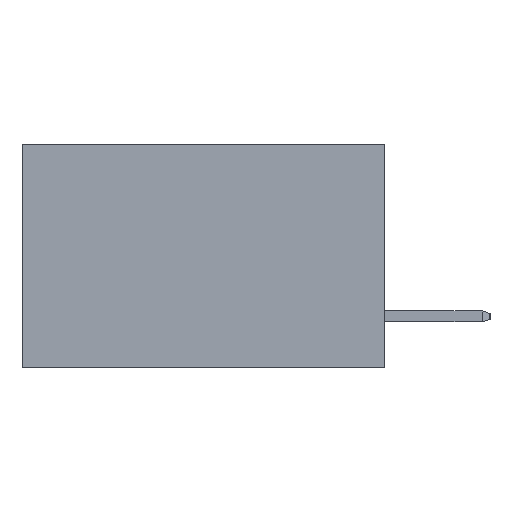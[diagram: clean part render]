
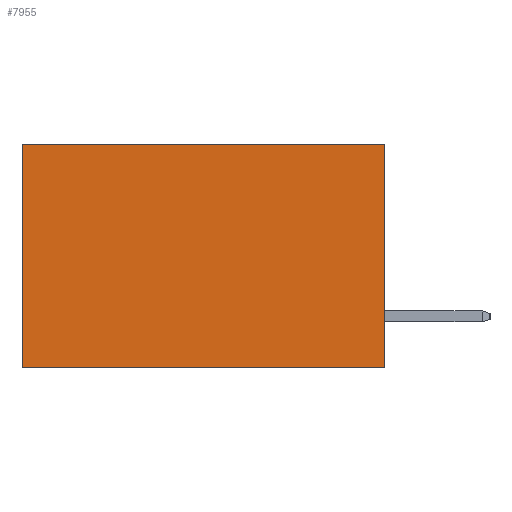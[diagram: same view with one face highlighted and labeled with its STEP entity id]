
A CAD part, left-side view. The second image highlights one B-rep face of the part: STEP entity #7955.
In plain terms, the highlighted planar face has unit normal (-1, 0, 0).
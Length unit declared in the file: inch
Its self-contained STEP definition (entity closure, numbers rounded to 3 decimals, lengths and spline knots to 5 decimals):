
#215 = DIRECTION ( 'NONE',  ( 0., 0., -1. ) ) ;
#793 = VECTOR ( 'NONE', #8180, 39.37008 ) ;
#795 = DIRECTION ( 'NONE',  ( 0., 1., 0. ) ) ;
#857 = CARTESIAN_POINT ( 'NONE',  ( 0.298, 0.6, 0. ) ) ;
#1012 = CARTESIAN_POINT ( 'NONE',  ( 0.298, 0., 0. ) ) ;
#2100 = VERTEX_POINT ( 'NONE', #857 ) ;
#3639 = VECTOR ( 'NONE', #14425, 39.37008 ) ;
#4481 = EDGE_CURVE ( 'NONE', #14590, #7413, #9179, .T. ) ;
#4878 = ORIENTED_EDGE ( 'NONE', *, *, #12892, .T. ) ;
#6045 = DIRECTION ( 'NONE',  ( 0., 0., -1. ) ) ;
#7413 = VERTEX_POINT ( 'NONE', #7998 ) ;
#7688 = PLANE ( 'NONE',  #20466 ) ;
#7955 = ADVANCED_FACE ( 'NONE', ( #20539 ), #7688, .F. ) ;
#7998 = CARTESIAN_POINT ( 'NONE',  ( 0.298, 0.6, -0.37 ) ) ;
#8180 = DIRECTION ( 'NONE',  ( 0., 1., 0. ) ) ;
#8559 = EDGE_CURVE ( 'NONE', #12378, #14590, #16873, .T. ) ;
#8561 = CARTESIAN_POINT ( 'NONE',  ( 0.298, 0.6, 0. ) ) ;
#9179 = LINE ( 'NONE', #16000, #793 ) ;
#9947 = EDGE_CURVE ( 'NONE', #12378, #2100, #10416, .T. ) ;
#10059 = CARTESIAN_POINT ( 'NONE',  ( 0.298, 0., -0.37 ) ) ;
#10416 = LINE ( 'NONE', #12481, #18530 ) ;
#10504 = EDGE_LOOP ( 'NONE', ( #4878, #12706, #16065, #16724 ) ) ;
#11179 = CARTESIAN_POINT ( 'NONE',  ( 0.298, 0., 0. ) ) ;
#11572 = LINE ( 'NONE', #8561, #19607 ) ;
#12378 = VERTEX_POINT ( 'NONE', #15541 ) ;
#12481 = CARTESIAN_POINT ( 'NONE',  ( 0.298, 0., 0. ) ) ;
#12706 = ORIENTED_EDGE ( 'NONE', *, *, #4481, .F. ) ;
#12892 = EDGE_CURVE ( 'NONE', #2100, #7413, #11572, .T. ) ;
#14425 = DIRECTION ( 'NONE',  ( 0., 0., -1. ) ) ;
#14590 = VERTEX_POINT ( 'NONE', #10059 ) ;
#15541 = CARTESIAN_POINT ( 'NONE',  ( 0.298, 0., 0. ) ) ;
#15951 = DIRECTION ( 'NONE',  ( 1., 0., 0. ) ) ;
#16000 = CARTESIAN_POINT ( 'NONE',  ( 0.298, 0., -0.37 ) ) ;
#16065 = ORIENTED_EDGE ( 'NONE', *, *, #8559, .F. ) ;
#16724 = ORIENTED_EDGE ( 'NONE', *, *, #9947, .T. ) ;
#16873 = LINE ( 'NONE', #11179, #3639 ) ;
#18530 = VECTOR ( 'NONE', #795, 39.37008 ) ;
#19607 = VECTOR ( 'NONE', #215, 39.37008 ) ;
#20466 = AXIS2_PLACEMENT_3D ( 'NONE', #1012, #15951, #6045 ) ;
#20539 = FACE_OUTER_BOUND ( 'NONE', #10504, .T. ) ;
